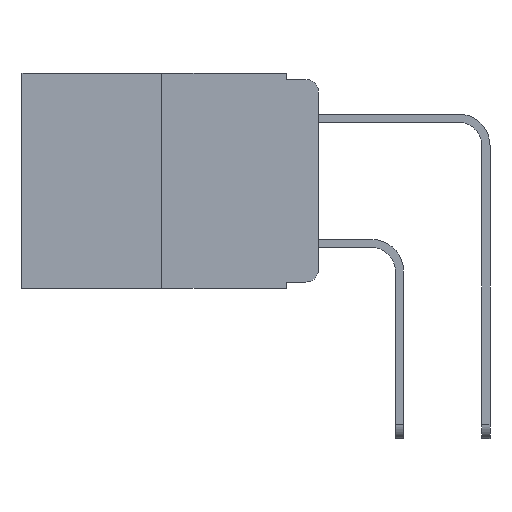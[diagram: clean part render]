
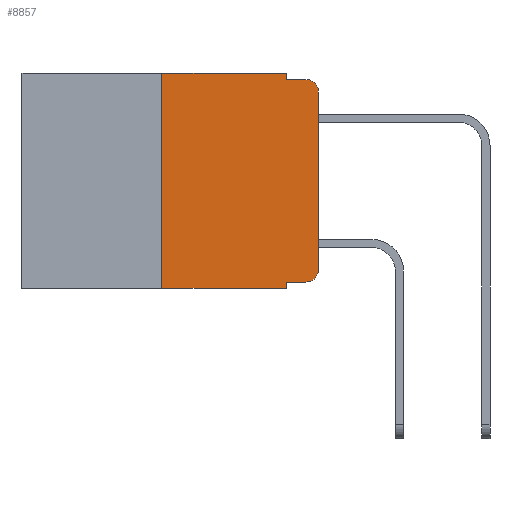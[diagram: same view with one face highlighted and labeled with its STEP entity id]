
A CAD part, left-side view. The second image highlights one B-rep face of the part: STEP entity #8857.
In plain terms, the highlighted planar face has unit normal (-1, 0, 0).
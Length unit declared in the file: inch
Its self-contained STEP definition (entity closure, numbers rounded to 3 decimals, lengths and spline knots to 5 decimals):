
#108 = EDGE_CURVE ( 'NONE', #551, #10913, #4959, .T. ) ;
#503 = EDGE_CURVE ( 'NONE', #4010, #4103, #3657, .T. ) ;
#524 = CARTESIAN_POINT ( 'NONE',  ( 0., 0.02, -0.313 ) ) ;
#551 = VERTEX_POINT ( 'NONE', #9424 ) ;
#1314 = LINE ( 'NONE', #6231, #7210 ) ;
#1344 = ORIENTED_EDGE ( 'NONE', *, *, #10209, .T. ) ;
#1522 = DIRECTION ( 'NONE',  ( 0., 0., -1. ) ) ;
#1587 = AXIS2_PLACEMENT_3D ( 'NONE', #13107, #14205, #7367 ) ;
#1705 = DIRECTION ( 'NONE',  ( 0., 0., -1. ) ) ;
#1798 = VECTOR ( 'NONE', #3438, 39.37008 ) ;
#1817 = CARTESIAN_POINT ( 'NONE',  ( 0., 0.051, 0. ) ) ;
#1890 = CARTESIAN_POINT ( 'NONE',  ( 0., 0.051, -0.333 ) ) ;
#2036 = ORIENTED_EDGE ( 'NONE', *, *, #14779, .F. ) ;
#2076 = EDGE_CURVE ( 'NONE', #3510, #4103, #13293, .T. ) ;
#2416 = CARTESIAN_POINT ( 'NONE',  ( 0., 0., -0.313 ) ) ;
#2597 = CARTESIAN_POINT ( 'NONE',  ( 0., 0.051, -0.333 ) ) ;
#2628 = VERTEX_POINT ( 'NONE', #13654 ) ;
#2767 = DIRECTION ( 'NONE',  ( 0., -1., 0. ) ) ;
#2805 = VERTEX_POINT ( 'NONE', #11735 ) ;
#2859 = EDGE_CURVE ( 'NONE', #10606, #3510, #15029, .T. ) ;
#2868 = AXIS2_PLACEMENT_3D ( 'NONE', #10840, #3877, #12019 ) ;
#3281 = VECTOR ( 'NONE', #12484, 39.37008 ) ;
#3412 = LINE ( 'NONE', #1817, #9638 ) ;
#3438 = DIRECTION ( 'NONE',  ( 0., 0., 1. ) ) ;
#3510 = VERTEX_POINT ( 'NONE', #4893 ) ;
#3657 = LINE ( 'NONE', #10046, #3281 ) ;
#3711 = ORIENTED_EDGE ( 'NONE', *, *, #2076, .T. ) ;
#3877 = DIRECTION ( 'NONE',  ( -1., 0., 0. ) ) ;
#4010 = VERTEX_POINT ( 'NONE', #4039 ) ;
#4039 = CARTESIAN_POINT ( 'NONE',  ( 0., 0.051, -0.01 ) ) ;
#4103 = VERTEX_POINT ( 'NONE', #12332 ) ;
#4190 = LINE ( 'NONE', #8146, #1798 ) ;
#4256 = DIRECTION ( 'NONE',  ( 0., -1., 0. ) ) ;
#4867 = DIRECTION ( 'NONE',  ( 0., 0., 1. ) ) ;
#4893 = CARTESIAN_POINT ( 'NONE',  ( 0., 0., -0.03 ) ) ;
#4959 = LINE ( 'NONE', #10752, #5325 ) ;
#5001 = PLANE ( 'NONE',  #1587 ) ;
#5075 = AXIS2_PLACEMENT_3D ( 'NONE', #524, #8750, #1705 ) ;
#5325 = VECTOR ( 'NONE', #6912, 39.37008 ) ;
#6005 = CARTESIAN_POINT ( 'NONE',  ( 0., 0., 0. ) ) ;
#6231 = CARTESIAN_POINT ( 'NONE',  ( 0., 0.051, 0. ) ) ;
#6483 = ORIENTED_EDGE ( 'NONE', *, *, #2859, .T. ) ;
#6912 = DIRECTION ( 'NONE',  ( 0., -1., 0. ) ) ;
#7061 = VERTEX_POINT ( 'NONE', #7268 ) ;
#7210 = VECTOR ( 'NONE', #1522, 39.37008 ) ;
#7268 = CARTESIAN_POINT ( 'NONE',  ( 0., 0.02, -0.333 ) ) ;
#7367 = DIRECTION ( 'NONE',  ( 0., 0., -1. ) ) ;
#8146 = CARTESIAN_POINT ( 'NONE',  ( 0., 0.25, 0. ) ) ;
#8750 = DIRECTION ( 'NONE',  ( -1., 0., 0. ) ) ;
#8857 = ADVANCED_FACE ( 'NONE', ( #14263 ), #5001, .F. ) ;
#8876 = VECTOR ( 'NONE', #4256, 39.37008 ) ;
#9424 = CARTESIAN_POINT ( 'NONE',  ( 0., 0.25, 0. ) ) ;
#9638 = VECTOR ( 'NONE', #9991, 39.37008 ) ;
#9965 = CARTESIAN_POINT ( 'NONE',  ( 0., 0.051, 0. ) ) ;
#9991 = DIRECTION ( 'NONE',  ( 0., 0., -1. ) ) ;
#10046 = CARTESIAN_POINT ( 'NONE',  ( 0., 0.051, -0.01 ) ) ;
#10058 = VERTEX_POINT ( 'NONE', #2597 ) ;
#10103 = LINE ( 'NONE', #14359, #12455 ) ;
#10106 = ORIENTED_EDGE ( 'NONE', *, *, #11186, .T. ) ;
#10209 = EDGE_CURVE ( 'NONE', #7061, #10606, #10852, .T. ) ;
#10606 = VERTEX_POINT ( 'NONE', #2416 ) ;
#10752 = CARTESIAN_POINT ( 'NONE',  ( 0., 0.473, 0. ) ) ;
#10840 = CARTESIAN_POINT ( 'NONE',  ( 0., 0.02, -0.03 ) ) ;
#10852 = CIRCLE ( 'NONE', #5075, 0.02 ) ;
#10913 = VERTEX_POINT ( 'NONE', #9965 ) ;
#10977 = EDGE_CURVE ( 'NONE', #10058, #7061, #12288, .T. ) ;
#11186 = EDGE_CURVE ( 'NONE', #2628, #2805, #10103, .T. ) ;
#11301 = VECTOR ( 'NONE', #4867, 39.37008 ) ;
#11735 = CARTESIAN_POINT ( 'NONE',  ( 0., 0.051, -0.343 ) ) ;
#11770 = EDGE_CURVE ( 'NONE', #10058, #2805, #1314, .T. ) ;
#11920 = ORIENTED_EDGE ( 'NONE', *, *, #108, .F. ) ;
#12019 = DIRECTION ( 'NONE',  ( 0., 0., -1. ) ) ;
#12288 = LINE ( 'NONE', #1890, #8876 ) ;
#12332 = CARTESIAN_POINT ( 'NONE',  ( 0., 0.02, -0.01 ) ) ;
#12455 = VECTOR ( 'NONE', #2767, 39.37008 ) ;
#12484 = DIRECTION ( 'NONE',  ( 0., -1., 0. ) ) ;
#12650 = ORIENTED_EDGE ( 'NONE', *, *, #13289, .F. ) ;
#13107 = CARTESIAN_POINT ( 'NONE',  ( 0., 0.473, 0. ) ) ;
#13289 = EDGE_CURVE ( 'NONE', #2628, #551, #4190, .T. ) ;
#13293 = CIRCLE ( 'NONE', #2868, 0.02 ) ;
#13320 = ORIENTED_EDGE ( 'NONE', *, *, #503, .F. ) ;
#13503 = ORIENTED_EDGE ( 'NONE', *, *, #11770, .F. ) ;
#13610 = EDGE_LOOP ( 'NONE', ( #6483, #3711, #13320, #2036, #11920, #12650, #10106, #13503, #14567, #1344 ) ) ;
#13654 = CARTESIAN_POINT ( 'NONE',  ( 0., 0.25, -0.343 ) ) ;
#14205 = DIRECTION ( 'NONE',  ( 1., 0., 0. ) ) ;
#14263 = FACE_OUTER_BOUND ( 'NONE', #13610, .T. ) ;
#14359 = CARTESIAN_POINT ( 'NONE',  ( 0., 0.473, -0.343 ) ) ;
#14567 = ORIENTED_EDGE ( 'NONE', *, *, #10977, .T. ) ;
#14779 = EDGE_CURVE ( 'NONE', #10913, #4010, #3412, .T. ) ;
#15029 = LINE ( 'NONE', #6005, #11301 ) ;
